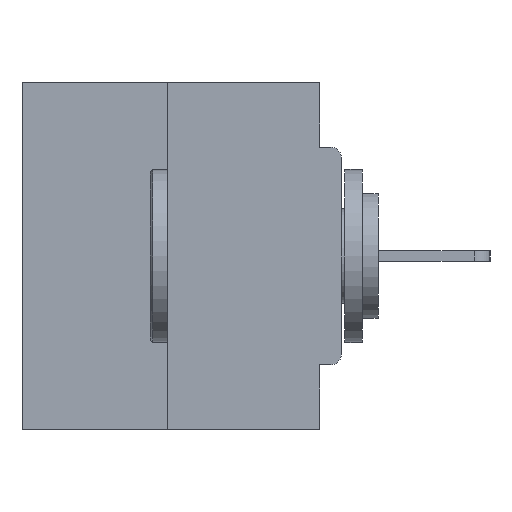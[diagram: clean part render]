
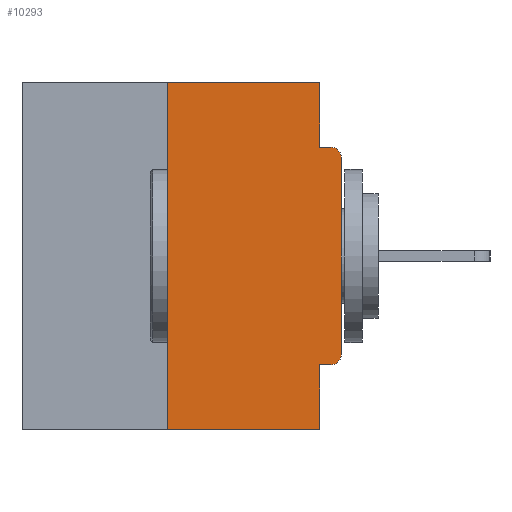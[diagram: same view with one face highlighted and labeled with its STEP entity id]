
A CAD part, left-side view. The second image highlights one B-rep face of the part: STEP entity #10293.
In plain terms, the highlighted planar face has unit normal (-1, 0, 0).
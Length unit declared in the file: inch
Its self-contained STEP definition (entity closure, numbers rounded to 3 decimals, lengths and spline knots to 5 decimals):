
#384 = VERTEX_POINT ( 'NONE', #19689 ) ;
#750 = CARTESIAN_POINT ( 'NONE',  ( 0., 0.25, 0. ) ) ;
#846 = DIRECTION ( 'NONE',  ( 0., 0., 1. ) ) ;
#857 = CARTESIAN_POINT ( 'NONE',  ( 0., 0.031, 0. ) ) ;
#987 = LINE ( 'NONE', #20792, #31166 ) ;
#1516 = VERTEX_POINT ( 'NONE', #37562 ) ;
#1600 = VERTEX_POINT ( 'NONE', #36753 ) ;
#1802 = VERTEX_POINT ( 'NONE', #16145 ) ;
#1868 = CARTESIAN_POINT ( 'NONE',  ( 0., 0.031, -0.4065 ) ) ;
#3323 = CARTESIAN_POINT ( 'NONE',  ( 0., 0.46, -0.5 ) ) ;
#4087 = CARTESIAN_POINT ( 'NONE',  ( 0., 0.25, 0. ) ) ;
#4132 = DIRECTION ( 'NONE',  ( 0., -1., 0. ) ) ;
#4508 = LINE ( 'NONE', #750, #33572 ) ;
#4684 = VECTOR ( 'NONE', #4132, 39.37008 ) ;
#5753 = EDGE_CURVE ( 'NONE', #1516, #8457, #28042, .T. ) ;
#6361 = DIRECTION ( 'NONE',  ( 0., -1., 0. ) ) ;
#7165 = CARTESIAN_POINT ( 'NONE',  ( 0., 0.46, 0. ) ) ;
#7417 = VECTOR ( 'NONE', #6361, 39.37008 ) ;
#7747 = LINE ( 'NONE', #857, #15684 ) ;
#8457 = VERTEX_POINT ( 'NONE', #22630 ) ;
#8628 = EDGE_CURVE ( 'NONE', #25530, #1600, #16276, .T. ) ;
#9861 = CARTESIAN_POINT ( 'NONE',  ( 0., 0.031, 0. ) ) ;
#10293 = ADVANCED_FACE ( 'NONE', ( #35781 ), #16421, .F. ) ;
#11141 = CARTESIAN_POINT ( 'NONE',  ( 0., 0., -0.0935 ) ) ;
#11192 = ORIENTED_EDGE ( 'NONE', *, *, #15282, .T. ) ;
#11793 = CARTESIAN_POINT ( 'NONE',  ( 0., 0.46, 0. ) ) ;
#12074 = DIRECTION ( 'NONE',  ( 0., 1., 0. ) ) ;
#12853 = CARTESIAN_POINT ( 'NONE',  ( 0., 0., 0. ) ) ;
#12914 = DIRECTION ( 'NONE',  ( -1., 0., 0. ) ) ;
#13487 = VECTOR ( 'NONE', #21152, 39.37008 ) ;
#13961 = LINE ( 'NONE', #11141, #14876 ) ;
#14742 = DIRECTION ( 'NONE',  ( 0., 0., -1. ) ) ;
#14876 = VECTOR ( 'NONE', #31285, 39.37008 ) ;
#15186 = DIRECTION ( 'NONE',  ( -1., 0., 0. ) ) ;
#15282 = EDGE_CURVE ( 'NONE', #1802, #1516, #26171, .T. ) ;
#15386 = ORIENTED_EDGE ( 'NONE', *, *, #24540, .F. ) ;
#15679 = DIRECTION ( 'NONE',  ( 0., 0., -1. ) ) ;
#15684 = VECTOR ( 'NONE', #15679, 39.37008 ) ;
#16090 = EDGE_CURVE ( 'NONE', #23433, #1600, #28757, .T. ) ;
#16145 = CARTESIAN_POINT ( 'NONE',  ( 0., 0.015, -0.4065 ) ) ;
#16276 = LINE ( 'NONE', #3323, #7417 ) ;
#16285 = ORIENTED_EDGE ( 'NONE', *, *, #28670, .F. ) ;
#16395 = EDGE_LOOP ( 'NONE', ( #19857, #24741, #21293, #23084, #16285, #11192, #19914, #36820, #35489, #15386 ) ) ;
#16421 = PLANE ( 'NONE',  #17340 ) ;
#17340 = AXIS2_PLACEMENT_3D ( 'NONE', #11793, #31892, #14742 ) ;
#17632 = CARTESIAN_POINT ( 'NONE',  ( 0., 0.25, -0.5 ) ) ;
#19685 = CARTESIAN_POINT ( 'NONE',  ( 0., 0.015, -0.0935 ) ) ;
#19689 = CARTESIAN_POINT ( 'NONE',  ( 0., 0.031, -0.0935 ) ) ;
#19857 = ORIENTED_EDGE ( 'NONE', *, *, #29437, .F. ) ;
#19914 = ORIENTED_EDGE ( 'NONE', *, *, #5753, .T. ) ;
#20536 = VECTOR ( 'NONE', #846, 39.37008 ) ;
#20792 = CARTESIAN_POINT ( 'NONE',  ( 0., 0., -0.4065 ) ) ;
#20988 = CIRCLE ( 'NONE', #35072, 0.015 ) ;
#21152 = DIRECTION ( 'NONE',  ( 0., 0., -1. ) ) ;
#21293 = ORIENTED_EDGE ( 'NONE', *, *, #8628, .T. ) ;
#22194 = VERTEX_POINT ( 'NONE', #4087 ) ;
#22630 = CARTESIAN_POINT ( 'NONE',  ( 0., 0., -0.1085 ) ) ;
#22875 = EDGE_CURVE ( 'NONE', #384, #25381, #13961, .T. ) ;
#23084 = ORIENTED_EDGE ( 'NONE', *, *, #16090, .F. ) ;
#23433 = VERTEX_POINT ( 'NONE', #1868 ) ;
#24004 = CARTESIAN_POINT ( 'NONE',  ( 0., 0.031, -0.5 ) ) ;
#24413 = DIRECTION ( 'NONE',  ( 0., 0., 1. ) ) ;
#24540 = EDGE_CURVE ( 'NONE', #35593, #384, #7747, .T. ) ;
#24741 = ORIENTED_EDGE ( 'NONE', *, *, #36210, .F. ) ;
#25381 = VERTEX_POINT ( 'NONE', #19685 ) ;
#25530 = VERTEX_POINT ( 'NONE', #17632 ) ;
#26171 = CIRCLE ( 'NONE', #28193, 0.015 ) ;
#27985 = LINE ( 'NONE', #7165, #4684 ) ;
#28042 = LINE ( 'NONE', #12853, #20536 ) ;
#28193 = AXIS2_PLACEMENT_3D ( 'NONE', #30097, #12914, #32954 ) ;
#28670 = EDGE_CURVE ( 'NONE', #1802, #23433, #987, .T. ) ;
#28757 = LINE ( 'NONE', #24004, #13487 ) ;
#29437 = EDGE_CURVE ( 'NONE', #22194, #35593, #27985, .T. ) ;
#30097 = CARTESIAN_POINT ( 'NONE',  ( 0., 0.015, -0.3915 ) ) ;
#31166 = VECTOR ( 'NONE', #12074, 39.37008 ) ;
#31285 = DIRECTION ( 'NONE',  ( 0., -1., 0. ) ) ;
#31892 = DIRECTION ( 'NONE',  ( 1., 0., 0. ) ) ;
#32325 = CARTESIAN_POINT ( 'NONE',  ( 0., 0.015, -0.1085 ) ) ;
#32755 = EDGE_CURVE ( 'NONE', #8457, #25381, #20988, .T. ) ;
#32954 = DIRECTION ( 'NONE',  ( 0., 0., -1. ) ) ;
#33572 = VECTOR ( 'NONE', #24413, 39.37008 ) ;
#35072 = AXIS2_PLACEMENT_3D ( 'NONE', #32325, #15186, #35163 ) ;
#35163 = DIRECTION ( 'NONE',  ( 0., 0., -1. ) ) ;
#35489 = ORIENTED_EDGE ( 'NONE', *, *, #22875, .F. ) ;
#35593 = VERTEX_POINT ( 'NONE', #9861 ) ;
#35781 = FACE_OUTER_BOUND ( 'NONE', #16395, .T. ) ;
#36210 = EDGE_CURVE ( 'NONE', #25530, #22194, #4508, .T. ) ;
#36753 = CARTESIAN_POINT ( 'NONE',  ( 0., 0.031, -0.5 ) ) ;
#36820 = ORIENTED_EDGE ( 'NONE', *, *, #32755, .T. ) ;
#37562 = CARTESIAN_POINT ( 'NONE',  ( 0., 0., -0.3915 ) ) ;
